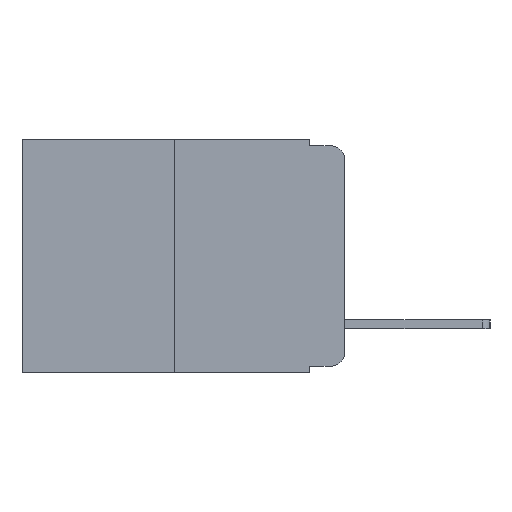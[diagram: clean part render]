
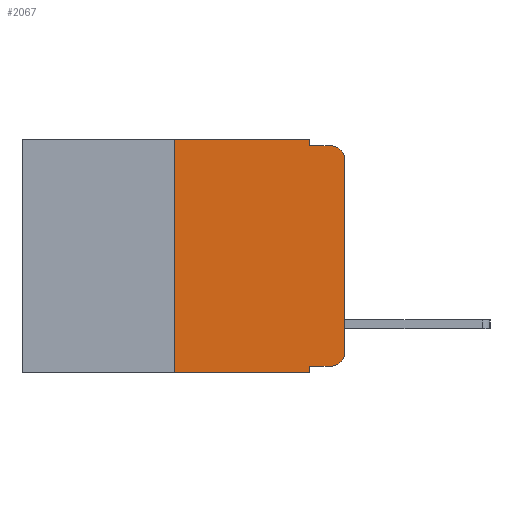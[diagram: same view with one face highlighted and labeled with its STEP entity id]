
A CAD part, left-side view. The second image highlights one B-rep face of the part: STEP entity #2067.
In plain terms, the highlighted planar face has unit normal (-1, 0, 0).
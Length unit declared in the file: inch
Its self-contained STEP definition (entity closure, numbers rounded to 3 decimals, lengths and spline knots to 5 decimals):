
#111 = ORIENTED_EDGE ( 'NONE', *, *, #3844, .F. ) ;
#161 = ORIENTED_EDGE ( 'NONE', *, *, #982, .F. ) ;
#527 = VERTEX_POINT ( 'NONE', #12027 ) ;
#731 = EDGE_CURVE ( 'NONE', #6462, #6083, #15212, .T. ) ;
#982 = EDGE_CURVE ( 'NONE', #6083, #5599, #8209, .T. ) ;
#1350 = VERTEX_POINT ( 'NONE', #9178 ) ;
#1421 = DIRECTION ( 'NONE',  ( 0., 0., -1. ) ) ;
#1499 = CARTESIAN_POINT ( 'NONE',  ( 0., 0.051, -0.01 ) ) ;
#1910 = DIRECTION ( 'NONE',  ( 1., 0., 0. ) ) ;
#2067 = ADVANCED_FACE ( 'NONE', ( #4010 ), #10269, .F. ) ;
#2286 = VECTOR ( 'NONE', #13566, 39.37008 ) ;
#2576 = DIRECTION ( 'NONE',  ( 0., -1., 0. ) ) ;
#2751 = VERTEX_POINT ( 'NONE', #7134 ) ;
#2824 = ORIENTED_EDGE ( 'NONE', *, *, #7455, .F. ) ;
#2882 = DIRECTION ( 'NONE',  ( -1., 0., 0. ) ) ;
#3148 = CARTESIAN_POINT ( 'NONE',  ( 0., 0.25, 0. ) ) ;
#3206 = DIRECTION ( 'NONE',  ( 0., 0., 1. ) ) ;
#3332 = EDGE_CURVE ( 'NONE', #14968, #5599, #8289, .T. ) ;
#3341 = VECTOR ( 'NONE', #9782, 39.37008 ) ;
#3434 = LINE ( 'NONE', #3148, #15203 ) ;
#3453 = EDGE_LOOP ( 'NONE', ( #5930, #6535, #161, #13121, #111, #2824, #12151, #6538, #9539, #9779 ) ) ;
#3764 = DIRECTION ( 'NONE',  ( 0., 0., -1. ) ) ;
#3844 = EDGE_CURVE ( 'NONE', #527, #6462, #9162, .T. ) ;
#3890 = CARTESIAN_POINT ( 'NONE',  ( 0., 0.051, -0.333 ) ) ;
#3992 = DIRECTION ( 'NONE',  ( 0., -1., 0. ) ) ;
#4010 = FACE_OUTER_BOUND ( 'NONE', #3453, .T. ) ;
#4168 = AXIS2_PLACEMENT_3D ( 'NONE', #14459, #1910, #3764 ) ;
#4356 = CARTESIAN_POINT ( 'NONE',  ( 0., 0.02, -0.01 ) ) ;
#4515 = LINE ( 'NONE', #13812, #8092 ) ;
#4553 = DIRECTION ( 'NONE',  ( 0., 0., 1. ) ) ;
#4790 = EDGE_CURVE ( 'NONE', #2751, #8237, #4515, .T. ) ;
#5599 = VERTEX_POINT ( 'NONE', #4356 ) ;
#5822 = DIRECTION ( 'NONE',  ( -1., 0., 0. ) ) ;
#5930 = ORIENTED_EDGE ( 'NONE', *, *, #10495, .T. ) ;
#6083 = VERTEX_POINT ( 'NONE', #12313 ) ;
#6419 = CARTESIAN_POINT ( 'NONE',  ( 0., 0., -0.313 ) ) ;
#6420 = VECTOR ( 'NONE', #1421, 39.37008 ) ;
#6462 = VERTEX_POINT ( 'NONE', #15218 ) ;
#6535 = ORIENTED_EDGE ( 'NONE', *, *, #3332, .T. ) ;
#6538 = ORIENTED_EDGE ( 'NONE', *, *, #4790, .F. ) ;
#7134 = CARTESIAN_POINT ( 'NONE',  ( 0., 0.051, -0.333 ) ) ;
#7244 = DIRECTION ( 'NONE',  ( 0., 0., -1. ) ) ;
#7455 = EDGE_CURVE ( 'NONE', #1350, #527, #3434, .T. ) ;
#7862 = VECTOR ( 'NONE', #2576, 39.37008 ) ;
#7901 = VERTEX_POINT ( 'NONE', #6419 ) ;
#8027 = CARTESIAN_POINT ( 'NONE',  ( 0., 0.051, -0.343 ) ) ;
#8092 = VECTOR ( 'NONE', #7244, 39.37008 ) ;
#8209 = LINE ( 'NONE', #1499, #7862 ) ;
#8237 = VERTEX_POINT ( 'NONE', #8027 ) ;
#8289 = CIRCLE ( 'NONE', #11482, 0.02 ) ;
#9162 = LINE ( 'NONE', #11404, #2286 ) ;
#9178 = CARTESIAN_POINT ( 'NONE',  ( 0., 0.25, -0.343 ) ) ;
#9539 = ORIENTED_EDGE ( 'NONE', *, *, #12991, .T. ) ;
#9634 = CARTESIAN_POINT ( 'NONE',  ( 0., 0.051, 0. ) ) ;
#9779 = ORIENTED_EDGE ( 'NONE', *, *, #11078, .T. ) ;
#9782 = DIRECTION ( 'NONE',  ( 0., -1., 0. ) ) ;
#10057 = CARTESIAN_POINT ( 'NONE',  ( 0., 0.02, -0.313 ) ) ;
#10260 = VERTEX_POINT ( 'NONE', #13323 ) ;
#10269 = PLANE ( 'NONE',  #4168 ) ;
#10379 = CARTESIAN_POINT ( 'NONE',  ( 0., 0., 0. ) ) ;
#10408 = LINE ( 'NONE', #3890, #3341 ) ;
#10495 = EDGE_CURVE ( 'NONE', #7901, #14968, #10595, .T. ) ;
#10595 = LINE ( 'NONE', #10379, #11946 ) ;
#10994 = EDGE_CURVE ( 'NONE', #1350, #8237, #13467, .T. ) ;
#11078 = EDGE_CURVE ( 'NONE', #10260, #7901, #15279, .T. ) ;
#11172 = DIRECTION ( 'NONE',  ( 0., 0., -1. ) ) ;
#11404 = CARTESIAN_POINT ( 'NONE',  ( 0., 0.473, 0. ) ) ;
#11482 = AXIS2_PLACEMENT_3D ( 'NONE', #12548, #5822, #13626 ) ;
#11929 = CARTESIAN_POINT ( 'NONE',  ( 0., 0., -0.03 ) ) ;
#11946 = VECTOR ( 'NONE', #4553, 39.37008 ) ;
#12027 = CARTESIAN_POINT ( 'NONE',  ( 0., 0.25, 0. ) ) ;
#12151 = ORIENTED_EDGE ( 'NONE', *, *, #10994, .T. ) ;
#12313 = CARTESIAN_POINT ( 'NONE',  ( 0., 0.051, -0.01 ) ) ;
#12548 = CARTESIAN_POINT ( 'NONE',  ( 0., 0.02, -0.03 ) ) ;
#12991 = EDGE_CURVE ( 'NONE', #2751, #10260, #10408, .T. ) ;
#13121 = ORIENTED_EDGE ( 'NONE', *, *, #731, .F. ) ;
#13126 = VECTOR ( 'NONE', #3992, 39.37008 ) ;
#13164 = CARTESIAN_POINT ( 'NONE',  ( 0., 0.473, -0.343 ) ) ;
#13323 = CARTESIAN_POINT ( 'NONE',  ( 0., 0.02, -0.333 ) ) ;
#13467 = LINE ( 'NONE', #13164, #13126 ) ;
#13566 = DIRECTION ( 'NONE',  ( 0., -1., 0. ) ) ;
#13626 = DIRECTION ( 'NONE',  ( 0., 0., -1. ) ) ;
#13812 = CARTESIAN_POINT ( 'NONE',  ( 0., 0.051, 0. ) ) ;
#14337 = AXIS2_PLACEMENT_3D ( 'NONE', #10057, #2882, #11172 ) ;
#14459 = CARTESIAN_POINT ( 'NONE',  ( 0., 0.473, 0. ) ) ;
#14968 = VERTEX_POINT ( 'NONE', #11929 ) ;
#15203 = VECTOR ( 'NONE', #3206, 39.37008 ) ;
#15212 = LINE ( 'NONE', #9634, #6420 ) ;
#15218 = CARTESIAN_POINT ( 'NONE',  ( 0., 0.051, 0. ) ) ;
#15279 = CIRCLE ( 'NONE', #14337, 0.02 ) ;
